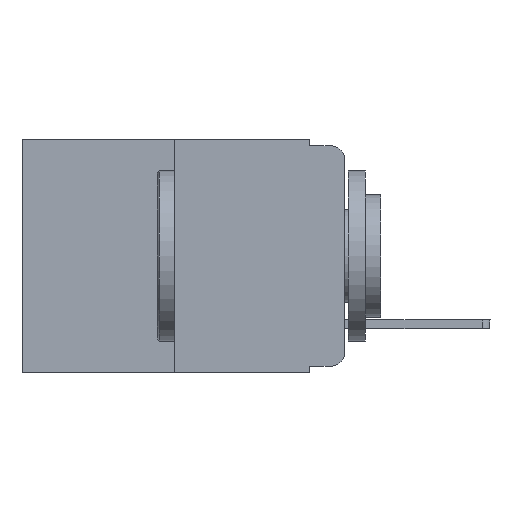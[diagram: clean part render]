
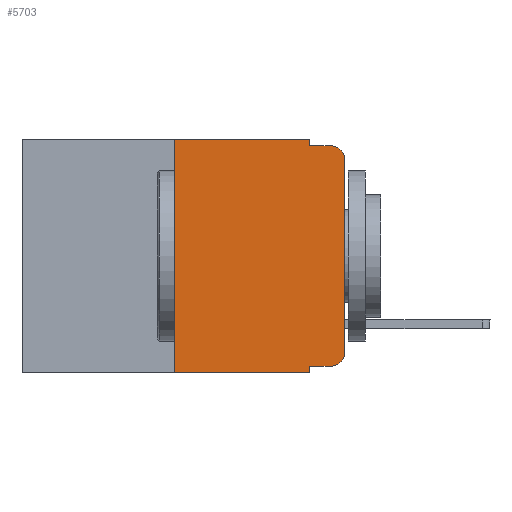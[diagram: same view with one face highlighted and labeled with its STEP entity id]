
A CAD part, left-side view. The second image highlights one B-rep face of the part: STEP entity #5703.
In plain terms, the highlighted planar face has unit normal (-1, 0, 0).
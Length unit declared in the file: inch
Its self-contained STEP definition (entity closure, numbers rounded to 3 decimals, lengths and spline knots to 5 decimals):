
#161 = CARTESIAN_POINT ( 'NONE',  ( 0., 0.25, -0.343 ) ) ;
#344 = ORIENTED_EDGE ( 'NONE', *, *, #11364, .T. ) ;
#368 = CARTESIAN_POINT ( 'NONE',  ( 0., 0.051, -0.333 ) ) ;
#425 = DIRECTION ( 'NONE',  ( 0., -1., 0. ) ) ;
#560 = LINE ( 'NONE', #2742, #9879 ) ;
#745 = LINE ( 'NONE', #2782, #12965 ) ;
#861 = VERTEX_POINT ( 'NONE', #6364 ) ;
#1010 = DIRECTION ( 'NONE',  ( 0., 0., -1. ) ) ;
#1147 = CARTESIAN_POINT ( 'NONE',  ( 0., 0.25, 0. ) ) ;
#1344 = VECTOR ( 'NONE', #1362, 39.37008 ) ;
#1353 = ORIENTED_EDGE ( 'NONE', *, *, #7337, .F. ) ;
#1358 = ORIENTED_EDGE ( 'NONE', *, *, #13160, .F. ) ;
#1362 = DIRECTION ( 'NONE',  ( 0., 0., 1. ) ) ;
#1730 = ORIENTED_EDGE ( 'NONE', *, *, #13992, .T. ) ;
#2080 = AXIS2_PLACEMENT_3D ( 'NONE', #11969, #2416, #1010 ) ;
#2416 = DIRECTION ( 'NONE',  ( -1., 0., 0. ) ) ;
#2592 = EDGE_LOOP ( 'NONE', ( #344, #10963, #1353, #17369, #12513, #1358, #7624, #5193, #7484, #1730 ) ) ;
#2742 = CARTESIAN_POINT ( 'NONE',  ( 0., 0.051, 0. ) ) ;
#2782 = CARTESIAN_POINT ( 'NONE',  ( 0., 0.473, -0.343 ) ) ;
#3139 = CARTESIAN_POINT ( 'NONE',  ( 0., 0.051, -0.333 ) ) ;
#3556 = VECTOR ( 'NONE', #14190, 39.37008 ) ;
#4155 = LINE ( 'NONE', #4855, #9565 ) ;
#4666 = VERTEX_POINT ( 'NONE', #13930 ) ;
#4737 = DIRECTION ( 'NONE',  ( 0., -1., 0. ) ) ;
#4855 = CARTESIAN_POINT ( 'NONE',  ( 0., 0.051, -0.01 ) ) ;
#5009 = LINE ( 'NONE', #7056, #1344 ) ;
#5193 = ORIENTED_EDGE ( 'NONE', *, *, #16028, .F. ) ;
#5216 = EDGE_CURVE ( 'NONE', #8078, #7108, #560, .T. ) ;
#5419 = DIRECTION ( 'NONE',  ( 0., -1., 0. ) ) ;
#5544 = DIRECTION ( 'NONE',  ( 0., 0., -1. ) ) ;
#5703 = ADVANCED_FACE ( 'NONE', ( #11637 ), #15429, .F. ) ;
#5734 = DIRECTION ( 'NONE',  ( 1., 0., 0. ) ) ;
#5863 = CARTESIAN_POINT ( 'NONE',  ( 0., 0.473, 0. ) ) ;
#5935 = VECTOR ( 'NONE', #425, 39.37008 ) ;
#6064 = CARTESIAN_POINT ( 'NONE',  ( 0., 0.051, -0.343 ) ) ;
#6362 = VERTEX_POINT ( 'NONE', #12288 ) ;
#6364 = CARTESIAN_POINT ( 'NONE',  ( 0., 0., -0.313 ) ) ;
#6489 = DIRECTION ( 'NONE',  ( 0., 0., -1. ) ) ;
#7038 = EDGE_CURVE ( 'NONE', #17525, #6362, #13785, .T. ) ;
#7056 = CARTESIAN_POINT ( 'NONE',  ( 0., 0., 0. ) ) ;
#7108 = VERTEX_POINT ( 'NONE', #9111 ) ;
#7197 = CARTESIAN_POINT ( 'NONE',  ( 0., 0.051, 0. ) ) ;
#7337 = EDGE_CURVE ( 'NONE', #7108, #6362, #4155, .T. ) ;
#7484 = ORIENTED_EDGE ( 'NONE', *, *, #16058, .T. ) ;
#7624 = ORIENTED_EDGE ( 'NONE', *, *, #16002, .T. ) ;
#7713 = AXIS2_PLACEMENT_3D ( 'NONE', #12084, #8077, #6489 ) ;
#7951 = AXIS2_PLACEMENT_3D ( 'NONE', #9736, #5734, #5544 ) ;
#8077 = DIRECTION ( 'NONE',  ( -1., 0., 0. ) ) ;
#8078 = VERTEX_POINT ( 'NONE', #13984 ) ;
#8479 = DIRECTION ( 'NONE',  ( 0., -1., 0. ) ) ;
#8787 = LINE ( 'NONE', #5863, #15369 ) ;
#9111 = CARTESIAN_POINT ( 'NONE',  ( 0., 0.051, -0.01 ) ) ;
#9278 = VECTOR ( 'NONE', #13590, 39.37008 ) ;
#9565 = VECTOR ( 'NONE', #4737, 39.37008 ) ;
#9736 = CARTESIAN_POINT ( 'NONE',  ( 0., 0.473, 0. ) ) ;
#9879 = VECTOR ( 'NONE', #15452, 39.37008 ) ;
#10963 = ORIENTED_EDGE ( 'NONE', *, *, #7038, .T. ) ;
#11364 = EDGE_CURVE ( 'NONE', #861, #17525, #5009, .T. ) ;
#11619 = VERTEX_POINT ( 'NONE', #14670 ) ;
#11633 = LINE ( 'NONE', #7197, #3556 ) ;
#11637 = FACE_OUTER_BOUND ( 'NONE', #2592, .T. ) ;
#11843 = CARTESIAN_POINT ( 'NONE',  ( 0., 0., -0.03 ) ) ;
#11969 = CARTESIAN_POINT ( 'NONE',  ( 0., 0.02, -0.03 ) ) ;
#12084 = CARTESIAN_POINT ( 'NONE',  ( 0., 0.02, -0.313 ) ) ;
#12176 = LINE ( 'NONE', #1147, #9278 ) ;
#12288 = CARTESIAN_POINT ( 'NONE',  ( 0., 0.02, -0.01 ) ) ;
#12513 = ORIENTED_EDGE ( 'NONE', *, *, #15434, .F. ) ;
#12965 = VECTOR ( 'NONE', #5419, 39.37008 ) ;
#13160 = EDGE_CURVE ( 'NONE', #14907, #4666, #12176, .T. ) ;
#13590 = DIRECTION ( 'NONE',  ( 0., 0., 1. ) ) ;
#13785 = CIRCLE ( 'NONE', #2080, 0.02 ) ;
#13895 = VERTEX_POINT ( 'NONE', #3139 ) ;
#13930 = CARTESIAN_POINT ( 'NONE',  ( 0., 0.25, 0. ) ) ;
#13984 = CARTESIAN_POINT ( 'NONE',  ( 0., 0.051, 0. ) ) ;
#13992 = EDGE_CURVE ( 'NONE', #11619, #861, #17310, .T. ) ;
#14190 = DIRECTION ( 'NONE',  ( 0., 0., -1. ) ) ;
#14670 = CARTESIAN_POINT ( 'NONE',  ( 0., 0.02, -0.333 ) ) ;
#14907 = VERTEX_POINT ( 'NONE', #161 ) ;
#15369 = VECTOR ( 'NONE', #8479, 39.37008 ) ;
#15429 = PLANE ( 'NONE',  #7951 ) ;
#15434 = EDGE_CURVE ( 'NONE', #4666, #8078, #8787, .T. ) ;
#15452 = DIRECTION ( 'NONE',  ( 0., 0., -1. ) ) ;
#16002 = EDGE_CURVE ( 'NONE', #14907, #16171, #745, .T. ) ;
#16028 = EDGE_CURVE ( 'NONE', #13895, #16171, #11633, .T. ) ;
#16058 = EDGE_CURVE ( 'NONE', #13895, #11619, #17020, .T. ) ;
#16171 = VERTEX_POINT ( 'NONE', #6064 ) ;
#17020 = LINE ( 'NONE', #368, #5935 ) ;
#17310 = CIRCLE ( 'NONE', #7713, 0.02 ) ;
#17369 = ORIENTED_EDGE ( 'NONE', *, *, #5216, .F. ) ;
#17525 = VERTEX_POINT ( 'NONE', #11843 ) ;
